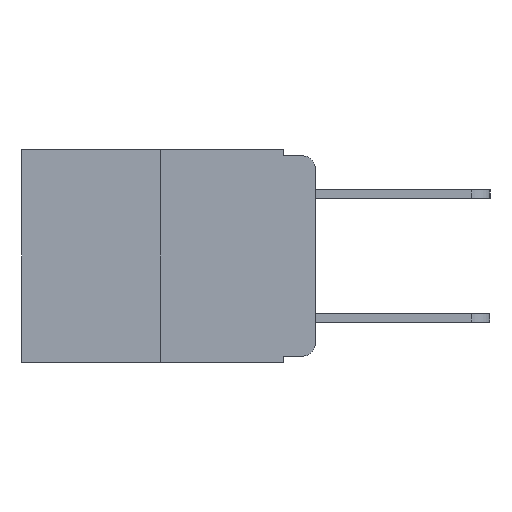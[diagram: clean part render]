
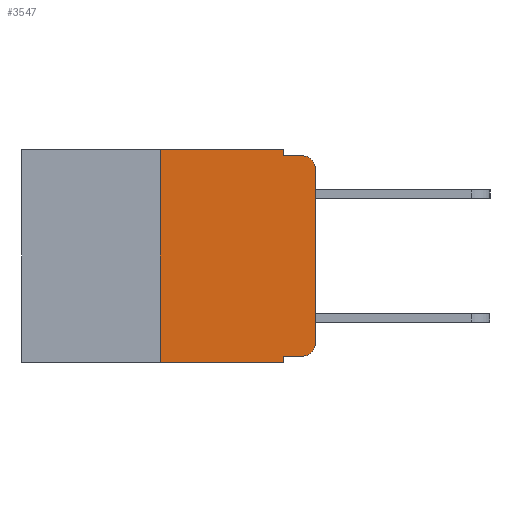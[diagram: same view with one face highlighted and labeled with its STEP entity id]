
A CAD part, left-side view. The second image highlights one B-rep face of the part: STEP entity #3547.
In plain terms, the highlighted planar face has unit normal (-1, 0, 0).
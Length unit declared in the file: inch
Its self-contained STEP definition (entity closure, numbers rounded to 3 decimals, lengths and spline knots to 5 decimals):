
#114 = VECTOR ( 'NONE', #17655, 39.37008 ) ;
#391 = CARTESIAN_POINT ( 'NONE',  ( 0., 0.051, 0. ) ) ;
#397 = VECTOR ( 'NONE', #8328, 39.37008 ) ;
#544 = EDGE_CURVE ( 'NONE', #11048, #4964, #12959, .T. ) ;
#938 = DIRECTION ( 'NONE',  ( -1., 0., 0. ) ) ;
#1251 = CARTESIAN_POINT ( 'NONE',  ( 0., 0.051, -0.333 ) ) ;
#1653 = LINE ( 'NONE', #391, #15927 ) ;
#1671 = PLANE ( 'NONE',  #14229 ) ;
#1911 = ORIENTED_EDGE ( 'NONE', *, *, #8311, .T. ) ;
#2446 = CIRCLE ( 'NONE', #4135, 0.02 ) ;
#2568 = VERTEX_POINT ( 'NONE', #12674 ) ;
#2678 = LINE ( 'NONE', #4332, #13325 ) ;
#2843 = CARTESIAN_POINT ( 'NONE',  ( 0., 0.25, 0. ) ) ;
#3015 = CARTESIAN_POINT ( 'NONE',  ( 0., 0.051, 0. ) ) ;
#3110 = VERTEX_POINT ( 'NONE', #9703 ) ;
#3494 = ORIENTED_EDGE ( 'NONE', *, *, #8161, .F. ) ;
#3547 = ADVANCED_FACE ( 'NONE', ( #14858 ), #1671, .F. ) ;
#3727 = DIRECTION ( 'NONE',  ( 0., 0., 1. ) ) ;
#3770 = CARTESIAN_POINT ( 'NONE',  ( 0., 0.25, -0.343 ) ) ;
#3973 = EDGE_LOOP ( 'NONE', ( #7273, #9467, #10980, #14149, #15579, #4286, #1911, #3494, #13619, #7914 ) ) ;
#4064 = EDGE_CURVE ( 'NONE', #6843, #4372, #14410, .T. ) ;
#4135 = AXIS2_PLACEMENT_3D ( 'NONE', #9473, #938, #10865 ) ;
#4230 = CARTESIAN_POINT ( 'NONE',  ( 0., 0.051, -0.333 ) ) ;
#4286 = ORIENTED_EDGE ( 'NONE', *, *, #4064, .F. ) ;
#4332 = CARTESIAN_POINT ( 'NONE',  ( 0., 0.473, 0. ) ) ;
#4372 = VERTEX_POINT ( 'NONE', #2843 ) ;
#4964 = VERTEX_POINT ( 'NONE', #14417 ) ;
#5106 = CARTESIAN_POINT ( 'NONE',  ( 0., 0.473, 0. ) ) ;
#5774 = DIRECTION ( 'NONE',  ( 0., -1., 0. ) ) ;
#6084 = AXIS2_PLACEMENT_3D ( 'NONE', #7971, #17256, #9329 ) ;
#6224 = DIRECTION ( 'NONE',  ( 0., 0., -1. ) ) ;
#6797 = EDGE_CURVE ( 'NONE', #4964, #9949, #16374, .T. ) ;
#6843 = VERTEX_POINT ( 'NONE', #3770 ) ;
#6893 = LINE ( 'NONE', #16885, #17517 ) ;
#7273 = ORIENTED_EDGE ( 'NONE', *, *, #544, .T. ) ;
#7388 = VERTEX_POINT ( 'NONE', #7466 ) ;
#7466 = CARTESIAN_POINT ( 'NONE',  ( 0., 0.051, -0.343 ) ) ;
#7914 = ORIENTED_EDGE ( 'NONE', *, *, #16004, .T. ) ;
#7971 = CARTESIAN_POINT ( 'NONE',  ( 0., 0.02, -0.03 ) ) ;
#8161 = EDGE_CURVE ( 'NONE', #11130, #7388, #16529, .T. ) ;
#8311 = EDGE_CURVE ( 'NONE', #6843, #7388, #6893, .T. ) ;
#8328 = DIRECTION ( 'NONE',  ( 0., 0., 1. ) ) ;
#8397 = EDGE_CURVE ( 'NONE', #3110, #2568, #1653, .T. ) ;
#8417 = CARTESIAN_POINT ( 'NONE',  ( 0., 0.051, -0.01 ) ) ;
#8727 = CARTESIAN_POINT ( 'NONE',  ( 0., 0.25, 0. ) ) ;
#9329 = DIRECTION ( 'NONE',  ( 0., 0., -1. ) ) ;
#9467 = ORIENTED_EDGE ( 'NONE', *, *, #6797, .T. ) ;
#9473 = CARTESIAN_POINT ( 'NONE',  ( 0., 0.02, -0.313 ) ) ;
#9703 = CARTESIAN_POINT ( 'NONE',  ( 0., 0.051, 0. ) ) ;
#9949 = VERTEX_POINT ( 'NONE', #16125 ) ;
#9970 = CARTESIAN_POINT ( 'NONE',  ( 0., 0., 0. ) ) ;
#10865 = DIRECTION ( 'NONE',  ( 0., 0., -1. ) ) ;
#10878 = CARTESIAN_POINT ( 'NONE',  ( 0., 0.02, -0.333 ) ) ;
#10980 = ORIENTED_EDGE ( 'NONE', *, *, #16126, .F. ) ;
#11048 = VERTEX_POINT ( 'NONE', #17469 ) ;
#11130 = VERTEX_POINT ( 'NONE', #4230 ) ;
#12158 = EDGE_CURVE ( 'NONE', #11130, #13098, #14779, .T. ) ;
#12237 = VECTOR ( 'NONE', #12722, 39.37008 ) ;
#12674 = CARTESIAN_POINT ( 'NONE',  ( 0., 0.051, -0.01 ) ) ;
#12722 = DIRECTION ( 'NONE',  ( 0., 0., -1. ) ) ;
#12949 = DIRECTION ( 'NONE',  ( 0., -1., 0. ) ) ;
#12959 = LINE ( 'NONE', #9970, #16447 ) ;
#13098 = VERTEX_POINT ( 'NONE', #10878 ) ;
#13325 = VECTOR ( 'NONE', #5774, 39.37008 ) ;
#13619 = ORIENTED_EDGE ( 'NONE', *, *, #12158, .T. ) ;
#14149 = ORIENTED_EDGE ( 'NONE', *, *, #8397, .F. ) ;
#14229 = AXIS2_PLACEMENT_3D ( 'NONE', #5106, #16729, #6224 ) ;
#14410 = LINE ( 'NONE', #8727, #397 ) ;
#14417 = CARTESIAN_POINT ( 'NONE',  ( 0., 0., -0.03 ) ) ;
#14779 = LINE ( 'NONE', #1251, #15187 ) ;
#14858 = FACE_OUTER_BOUND ( 'NONE', #3973, .T. ) ;
#15187 = VECTOR ( 'NONE', #17644, 39.37008 ) ;
#15579 = ORIENTED_EDGE ( 'NONE', *, *, #16185, .F. ) ;
#15927 = VECTOR ( 'NONE', #16994, 39.37008 ) ;
#16004 = EDGE_CURVE ( 'NONE', #13098, #11048, #2446, .T. ) ;
#16125 = CARTESIAN_POINT ( 'NONE',  ( 0., 0.02, -0.01 ) ) ;
#16126 = EDGE_CURVE ( 'NONE', #2568, #9949, #17581, .T. ) ;
#16185 = EDGE_CURVE ( 'NONE', #4372, #3110, #2678, .T. ) ;
#16374 = CIRCLE ( 'NONE', #6084, 0.02 ) ;
#16447 = VECTOR ( 'NONE', #3727, 39.37008 ) ;
#16529 = LINE ( 'NONE', #3015, #12237 ) ;
#16729 = DIRECTION ( 'NONE',  ( 1., 0., 0. ) ) ;
#16885 = CARTESIAN_POINT ( 'NONE',  ( 0., 0.473, -0.343 ) ) ;
#16994 = DIRECTION ( 'NONE',  ( 0., 0., -1. ) ) ;
#17256 = DIRECTION ( 'NONE',  ( -1., 0., 0. ) ) ;
#17469 = CARTESIAN_POINT ( 'NONE',  ( 0., 0., -0.313 ) ) ;
#17517 = VECTOR ( 'NONE', #12949, 39.37008 ) ;
#17581 = LINE ( 'NONE', #8417, #114 ) ;
#17644 = DIRECTION ( 'NONE',  ( 0., -1., 0. ) ) ;
#17655 = DIRECTION ( 'NONE',  ( 0., -1., 0. ) ) ;
